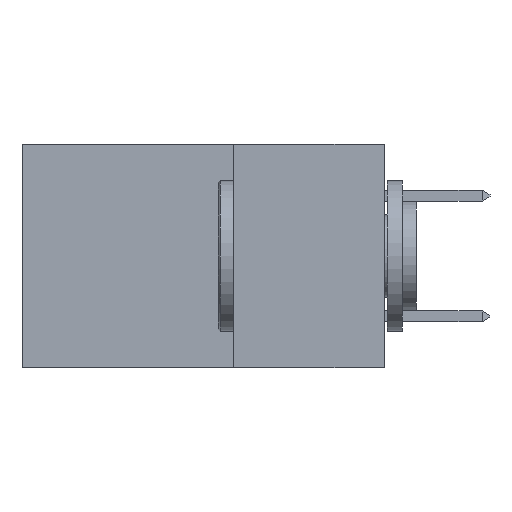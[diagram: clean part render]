
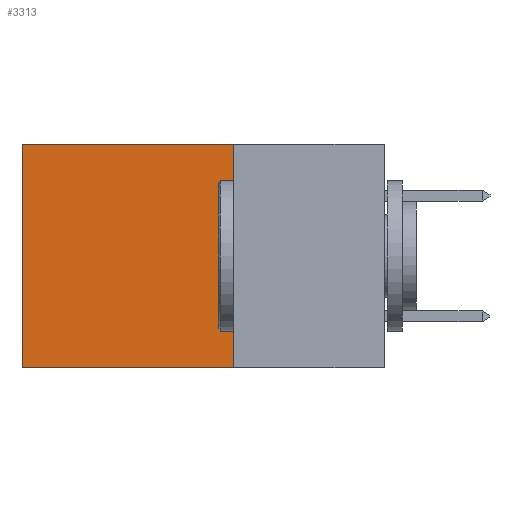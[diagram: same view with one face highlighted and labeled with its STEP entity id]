
A CAD part, left-side view. The second image highlights one B-rep face of the part: STEP entity #3313.
In plain terms, the highlighted planar face has unit normal (-1, 0, 0).
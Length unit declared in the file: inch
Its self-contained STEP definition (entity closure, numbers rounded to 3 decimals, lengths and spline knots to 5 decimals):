
#93 = ORIENTED_EDGE ( 'NONE', *, *, #4781, .T. ) ;
#485 = ORIENTED_EDGE ( 'NONE', *, *, #3448, .F. ) ;
#1212 = VERTEX_POINT ( 'NONE', #7258 ) ;
#1862 = VERTEX_POINT ( 'NONE', #5268 ) ;
#1893 = DIRECTION ( 'NONE',  ( 0., 0., -1. ) ) ;
#2048 = CARTESIAN_POINT ( 'NONE',  ( 0.2875, 0.25, 0. ) ) ;
#2193 = VECTOR ( 'NONE', #2443, 39.37008 ) ;
#2443 = DIRECTION ( 'NONE',  ( 0., 1., 0. ) ) ;
#2503 = CARTESIAN_POINT ( 'NONE',  ( 0.2875, 0.25, 0. ) ) ;
#2507 = DIRECTION ( 'NONE',  ( 0., 1., 0. ) ) ;
#2671 = CARTESIAN_POINT ( 'NONE',  ( 0.2875, 0.25, -0.37 ) ) ;
#2758 = DIRECTION ( 'NONE',  ( 1., 0., 0. ) ) ;
#2820 = PLANE ( 'NONE',  #5190 ) ;
#2823 = CARTESIAN_POINT ( 'NONE',  ( 0.2875, 0.25, 0. ) ) ;
#3172 = VERTEX_POINT ( 'NONE', #5260 ) ;
#3302 = EDGE_CURVE ( 'NONE', #4442, #3172, #6387, .T. ) ;
#3313 = ADVANCED_FACE ( 'NONE', ( #9497 ), #2820, .F. ) ;
#3448 = EDGE_CURVE ( 'NONE', #1212, #4442, #6675, .T. ) ;
#3455 = VECTOR ( 'NONE', #2507, 39.37008 ) ;
#3700 = DIRECTION ( 'NONE',  ( 0., 0., -1. ) ) ;
#3762 = CARTESIAN_POINT ( 'NONE',  ( 0.2875, 0.25, -0.37 ) ) ;
#4052 = ORIENTED_EDGE ( 'NONE', *, *, #6680, .T. ) ;
#4442 = VERTEX_POINT ( 'NONE', #3762 ) ;
#4775 = VECTOR ( 'NONE', #7694, 39.37008 ) ;
#4781 = EDGE_CURVE ( 'NONE', #1212, #1862, #5628, .T. ) ;
#5190 = AXIS2_PLACEMENT_3D ( 'NONE', #2823, #2758, #3700 ) ;
#5260 = CARTESIAN_POINT ( 'NONE',  ( 0.2875, 0.6, -0.37 ) ) ;
#5268 = CARTESIAN_POINT ( 'NONE',  ( 0.2875, 0.6, 0. ) ) ;
#5628 = LINE ( 'NONE', #2503, #3455 ) ;
#5784 = VECTOR ( 'NONE', #1893, 39.37008 ) ;
#6166 = ORIENTED_EDGE ( 'NONE', *, *, #3302, .F. ) ;
#6387 = LINE ( 'NONE', #2671, #2193 ) ;
#6573 = CARTESIAN_POINT ( 'NONE',  ( 0.2875, 0.6, 0. ) ) ;
#6675 = LINE ( 'NONE', #2048, #4775 ) ;
#6680 = EDGE_CURVE ( 'NONE', #1862, #3172, #9361, .T. ) ;
#7258 = CARTESIAN_POINT ( 'NONE',  ( 0.2875, 0.25, 0. ) ) ;
#7694 = DIRECTION ( 'NONE',  ( 0., 0., -1. ) ) ;
#9361 = LINE ( 'NONE', #6573, #5784 ) ;
#9497 = FACE_OUTER_BOUND ( 'NONE', #9565, .T. ) ;
#9565 = EDGE_LOOP ( 'NONE', ( #4052, #6166, #485, #93 ) ) ;
